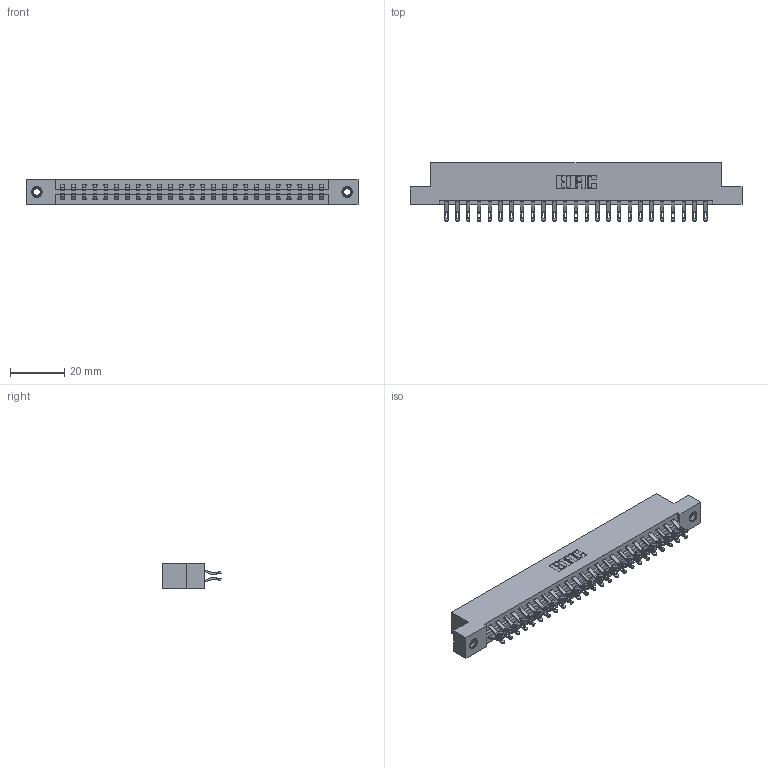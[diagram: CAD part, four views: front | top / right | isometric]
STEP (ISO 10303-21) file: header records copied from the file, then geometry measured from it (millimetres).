
FILE_DESCRIPTION (( 'STEP AP203' ), '1' );
FILE_NAME ('387-050-555-207.STEP', '2019-10-19T02:11:50', ( '' ), ( '' ), 'SwSTEP 2.0', 'SolidWorks 2016', '' );
FILE_SCHEMA (( 'CONFIG_CONTROL_DESIGN' ));
Length unit declared in the file: inch
Products named in the file (4): 387-050-555-207; 345-292-001_555 Tail; 345-250-001_345-250-005-103; 337 Part_Flush Mounting Lugs - 0.156 Dia-TI
Assembly tree (53 placements, depth 2):
  387-050-555-207
    337 Part_Flush Mounting Lugs - 0.156 Dia-TI
    345-292-001_555 Tail  x50
    345-250-001_345-250-005-103  x2
Bounding box: 122.07 x 21.47 x 9.4 mm (x, y, z)
Volume: 12770.2 mm3; surface area: 14854.1 mm2
Topology: 53 solids, 53 shells, 3174 faces, 9897 edges, 6590 vertices
Faces by surface type: plane 1902, cylinder 1256, cone 12, torus 4
Entity records: 23094 total; most frequent: CARTESIAN_POINT 3919, ORIENTED_EDGE 3818, DIRECTION 3367, EDGE_CURVE 1909, LINE 1741, VECTOR 1741, VERTEX_POINT 1268, AXIS2_PLACEMENT_3D 813
